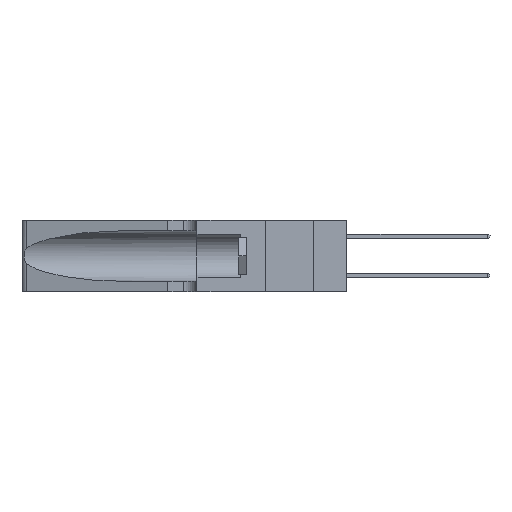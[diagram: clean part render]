
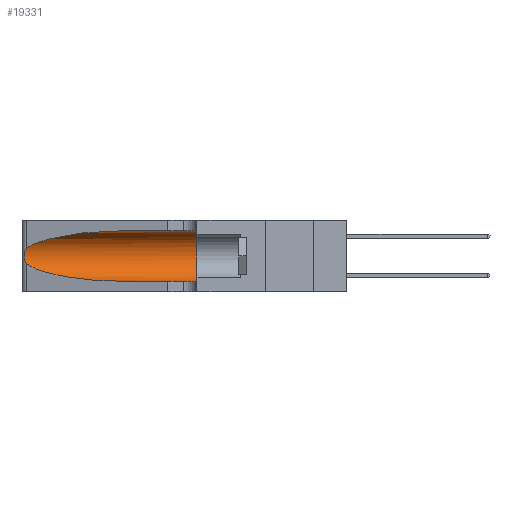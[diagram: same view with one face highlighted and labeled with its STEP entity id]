
A CAD part, left-side view. The second image highlights one B-rep face of the part: STEP entity #19331.
In plain terms, the highlighted cylindrical face has radius 3.308 mm (diameter 6.617 mm), a partial arc.
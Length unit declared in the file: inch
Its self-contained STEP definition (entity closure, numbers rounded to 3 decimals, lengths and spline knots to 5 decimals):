
#1396 = VERTEX_POINT ( 'NONE', #14793 ) ;
#2534 = VERTEX_POINT ( 'NONE', #26903 ) ;
#3075 = LINE ( 'NONE', #32126, #5923 ) ;
#3398 = CARTESIAN_POINT ( 'NONE',  ( 0.1305, 1.61858, 0.185 ) ) ;
#3518 = CARTESIAN_POINT ( 'NONE',  ( 0.1305, 0.35, 0.05475 ) ) ;
#3913 = CARTESIAN_POINT ( 'NONE',  ( 0.1305, 0.35, 0.185 ) ) ;
#4264 = ORIENTED_EDGE ( 'NONE', *, *, #24433, .T. ) ;
#4961 =( BOUNDED_CURVE ( )  B_SPLINE_CURVE ( 3, ( #29949, #14847, #32708, #23523 ),
 .UNSPECIFIED., .F., .T. ) 
 B_SPLINE_CURVE_WITH_KNOTS ( ( 4, 4 ),
 ( 1.5708, 2.84003 ),
 .UNSPECIFIED. ) 
 CURVE ( )  GEOMETRIC_REPRESENTATION_ITEM ( )  RATIONAL_B_SPLINE_CURVE ( ( 1., 0.87, 0.87, 1. ) ) 
 REPRESENTATION_ITEM ( '' )  );
#5556 = CARTESIAN_POINT ( 'NONE',  ( 0.1305, 0.72297, 0.05475 ) ) ;
#5923 = VECTOR ( 'NONE', #28844, 39.37008 ) ;
#6281 = CARTESIAN_POINT ( 'NONE',  ( 0.25555, 1.22994, 0.2215 ) ) ;
#6373 = EDGE_CURVE ( 'NONE', #1396, #32987, #34180, .T. ) ;
#6408 = CARTESIAN_POINT ( 'NONE',  ( 0.25789, 1.23486, 0.15765 ) ) ;
#6669 = CARTESIAN_POINT ( 'NONE',  ( 0.26075, 1.23896, 0.178 ) ) ;
#6929 = DIRECTION ( 'NONE',  ( 0., 1., 0. ) ) ;
#6947 = VERTEX_POINT ( 'NONE', #19197 ) ;
#7944 = CARTESIAN_POINT ( 'NONE',  ( 0.1305, 0.72297, 0.05475 ) ) ;
#8097 = EDGE_CURVE ( 'NONE', #2534, #6947, #31751, .T. ) ;
#8665 = ORIENTED_EDGE ( 'NONE', *, *, #6373, .T. ) ;
#9153 = ORIENTED_EDGE ( 'NONE', *, *, #29747, .T. ) ;
#9602 = CARTESIAN_POINT ( 'NONE',  ( 0.26017, 1.23833, 0.17102 ) ) ;
#9674 = EDGE_LOOP ( 'NONE', ( #9153, #24740, #8665, #4264, #22706, #23019 ) ) ;
#10016 = DIRECTION ( 'NONE',  ( 0., 0., 1. ) ) ;
#12385 = CARTESIAN_POINT ( 'NONE',  ( 0.25854, 1.2359, 0.20912 ) ) ;
#12624 = CARTESIAN_POINT ( 'NONE',  ( 0.25639, 1.23186, 0.15144 ) ) ;
#13667 = CARTESIAN_POINT ( 'NONE',  ( 0.18966, 0.96281, 0.05475 ) ) ;
#14203 = CARTESIAN_POINT ( 'NONE',  ( 0.2373, 1.15595, 0.08982 ) ) ;
#14793 = CARTESIAN_POINT ( 'NONE',  ( 0.25487, 1.22718, 0.14631 ) ) ;
#14847 = CARTESIAN_POINT ( 'NONE',  ( 0.18966, 0.96281, 0.31525 ) ) ;
#15566 = DIRECTION ( 'NONE',  ( 0., 0., -1. ) ) ;
#15833 = VERTEX_POINT ( 'NONE', #18663 ) ;
#18663 = CARTESIAN_POINT ( 'NONE',  ( 0.25487, 1.22718, 0.22369 ) ) ;
#19064 = AXIS2_PLACEMENT_3D ( 'NONE', #3398, #30544, #15566 ) ;
#19197 = CARTESIAN_POINT ( 'NONE',  ( 0.1305, 0.35, 0.31525 ) ) ;
#19331 = ADVANCED_FACE ( 'NONE', ( #29928 ), #34117, .F. ) ;
#19388 = EDGE_CURVE ( 'NONE', #6947, #25781, #29447, .T. ) ;
#21476 = CARTESIAN_POINT ( 'NONE',  ( 0.26018, 1.23835, 0.19895 ) ) ;
#22691 = B_SPLINE_CURVE_WITH_KNOTS ( 'NONE', 3,
 ( #27649, #6281, #27405, #30525, #12385, #21476, #24491, #6669, #9602, #30654, #6408, #12624, #36562, #33655 ),
 .UNSPECIFIED., .F., .F.,
 ( 4, 2, 2, 2, 2, 2, 4 ),
 ( 0., 0.00027, 0.00053, 0.00107, 0.0016, 0.00187, 0.00214 ),
 .UNSPECIFIED. ) ;
#22706 = ORIENTED_EDGE ( 'NONE', *, *, #19388, .F. ) ;
#22815 = VECTOR ( 'NONE', #34354, 39.37008 ) ;
#23019 = ORIENTED_EDGE ( 'NONE', *, *, #8097, .F. ) ;
#23122 = CARTESIAN_POINT ( 'NONE',  ( 0.25487, 1.22718, 0.14631 ) ) ;
#23523 = CARTESIAN_POINT ( 'NONE',  ( 0.25487, 1.22718, 0.22369 ) ) ;
#24433 = EDGE_CURVE ( 'NONE', #32987, #25781, #3075, .T. ) ;
#24491 = CARTESIAN_POINT ( 'NONE',  ( 0.26075, 1.23896, 0.19203 ) ) ;
#24740 = ORIENTED_EDGE ( 'NONE', *, *, #34040, .T. ) ;
#25781 = VERTEX_POINT ( 'NONE', #3518 ) ;
#26903 = CARTESIAN_POINT ( 'NONE',  ( 0.1305, 0.72297, 0.31525 ) ) ;
#27405 = CARTESIAN_POINT ( 'NONE',  ( 0.25639, 1.23184, 0.21858 ) ) ;
#27649 = CARTESIAN_POINT ( 'NONE',  ( 0.25487, 1.22718, 0.22369 ) ) ;
#28844 = DIRECTION ( 'NONE',  ( 0., -1., 0. ) ) ;
#29447 = CIRCLE ( 'NONE', #31143, 0.13025 ) ;
#29747 = EDGE_CURVE ( 'NONE', #2534, #15833, #4961, .T. ) ;
#29928 = FACE_OUTER_BOUND ( 'NONE', #9674, .T. ) ;
#29949 = CARTESIAN_POINT ( 'NONE',  ( 0.1305, 0.72297, 0.31525 ) ) ;
#30525 = CARTESIAN_POINT ( 'NONE',  ( 0.25787, 1.23484, 0.2124 ) ) ;
#30544 = DIRECTION ( 'NONE',  ( 0., -1., 0. ) ) ;
#30654 = CARTESIAN_POINT ( 'NONE',  ( 0.25856, 1.23593, 0.16098 ) ) ;
#31143 = AXIS2_PLACEMENT_3D ( 'NONE', #3913, #6929, #10016 ) ;
#31751 = LINE ( 'NONE', #37122, #22815 ) ;
#32126 = CARTESIAN_POINT ( 'NONE',  ( 0.1305, 1.61858, 0.05475 ) ) ;
#32708 = CARTESIAN_POINT ( 'NONE',  ( 0.2373, 1.15595, 0.28018 ) ) ;
#32987 = VERTEX_POINT ( 'NONE', #7944 ) ;
#33655 = CARTESIAN_POINT ( 'NONE',  ( 0.25487, 1.22718, 0.14631 ) ) ;
#34040 = EDGE_CURVE ( 'NONE', #15833, #1396, #22691, .T. ) ;
#34117 = CYLINDRICAL_SURFACE ( 'NONE', #19064, 0.13025 ) ;
#34180 =( BOUNDED_CURVE ( )  B_SPLINE_CURVE ( 3, ( #23122, #14203, #13667, #5556 ),
 .UNSPECIFIED., .F., .F. ) 
 B_SPLINE_CURVE_WITH_KNOTS ( ( 4, 4 ),
 ( 3.44316, 4.71239 ),
 .UNSPECIFIED. ) 
 CURVE ( )  GEOMETRIC_REPRESENTATION_ITEM ( )  RATIONAL_B_SPLINE_CURVE ( ( 1., 0.87, 0.87, 1. ) ) 
 REPRESENTATION_ITEM ( '' )  );
#34354 = DIRECTION ( 'NONE',  ( 0., -1., 0. ) ) ;
#36562 = CARTESIAN_POINT ( 'NONE',  ( 0.25555, 1.22993, 0.14849 ) ) ;
#37122 = CARTESIAN_POINT ( 'NONE',  ( 0.1305, 1.61858, 0.31525 ) ) ;
